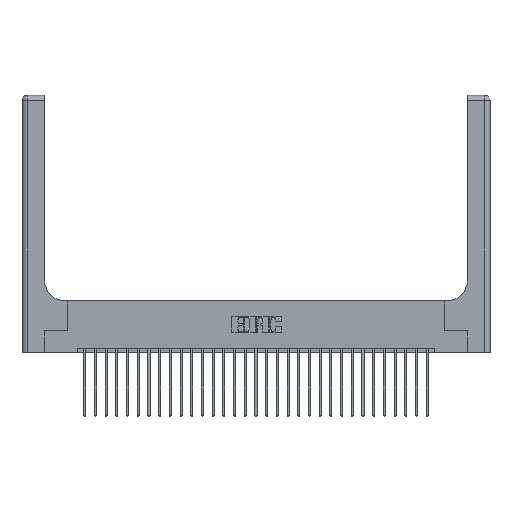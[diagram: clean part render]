
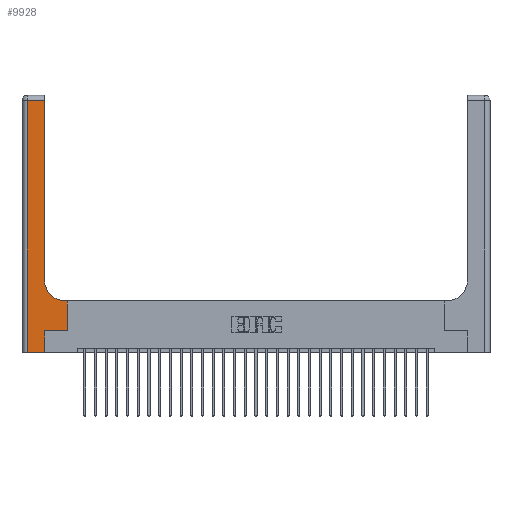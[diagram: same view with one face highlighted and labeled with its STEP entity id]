
A CAD part, top view. The second image highlights one B-rep face of the part: STEP entity #9928.
In plain terms, the highlighted planar face has unit normal (0, 0, 1).
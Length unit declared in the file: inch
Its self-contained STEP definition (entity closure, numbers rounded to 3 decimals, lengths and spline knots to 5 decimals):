
#800 = DIRECTION ( 'NONE',  ( 0., 1., 0. ) ) ;
#1074 = CARTESIAN_POINT ( 'NONE',  ( 0.51, 0.6, 0.37 ) ) ;
#1506 = ORIENTED_EDGE ( 'NONE', *, *, #21290, .T. ) ;
#2542 = CARTESIAN_POINT ( 'NONE',  ( 0.528, 0.25, 0.37 ) ) ;
#5061 = CARTESIAN_POINT ( 'NONE',  ( 0.51, 0.85, 0.37 ) ) ;
#5856 = CARTESIAN_POINT ( 'NONE',  ( 0., 0., 0.37 ) ) ;
#5992 = LINE ( 'NONE', #14007, #18834 ) ;
#6146 = DIRECTION ( 'NONE',  ( 1., 0., 0. ) ) ;
#6627 = ORIENTED_EDGE ( 'NONE', *, *, #27647, .T. ) ;
#6650 = DIRECTION ( 'NONE',  ( 0., 1., 0. ) ) ;
#7171 = VECTOR ( 'NONE', #800, 39.37008 ) ;
#7506 = CARTESIAN_POINT ( 'NONE',  ( 0.26, 2.94, 0.37 ) ) ;
#7764 = ORIENTED_EDGE ( 'NONE', *, *, #26584, .T. ) ;
#7914 = CARTESIAN_POINT ( 'NONE',  ( 0.06, 0., 0.37 ) ) ;
#8118 = DIRECTION ( 'NONE',  ( 0., 0., -1. ) ) ;
#9003 = CARTESIAN_POINT ( 'NONE',  ( 0.26, 3., 0.37 ) ) ;
#9518 = LINE ( 'NONE', #13401, #7171 ) ;
#9928 = ADVANCED_FACE ( 'NONE', ( #19745 ), #16728, .F. ) ;
#9992 = AXIS2_PLACEMENT_3D ( 'NONE', #23475, #8118, #25676 ) ;
#11056 = CARTESIAN_POINT ( 'NONE',  ( 0.265, 0.25, 0.37 ) ) ;
#11061 = VERTEX_POINT ( 'NONE', #2542 ) ;
#11272 = CARTESIAN_POINT ( 'NONE',  ( 0.528, 0.6, 0.37 ) ) ;
#11327 = ORIENTED_EDGE ( 'NONE', *, *, #14260, .T. ) ;
#11352 = CARTESIAN_POINT ( 'NONE',  ( 0.265, 0.25, 0.37 ) ) ;
#11726 = DIRECTION ( 'NONE',  ( 0., -1., 0. ) ) ;
#11970 = EDGE_CURVE ( 'NONE', #19686, #14375, #26737, .T. ) ;
#12166 = VERTEX_POINT ( 'NONE', #1074 ) ;
#13065 = ORIENTED_EDGE ( 'NONE', *, *, #27067, .T. ) ;
#13116 = VERTEX_POINT ( 'NONE', #19005 ) ;
#13401 = CARTESIAN_POINT ( 'NONE',  ( 0.528, 0.25, 0.37 ) ) ;
#13764 = DIRECTION ( 'NONE',  ( 1., 0., 0. ) ) ;
#13942 = LINE ( 'NONE', #11056, #23714 ) ;
#14007 = CARTESIAN_POINT ( 'NONE',  ( 0.06, 3., 0.37 ) ) ;
#14113 = VERTEX_POINT ( 'NONE', #27841 ) ;
#14260 = EDGE_CURVE ( 'NONE', #23562, #11061, #13942, .T. ) ;
#14375 = VERTEX_POINT ( 'NONE', #24067 ) ;
#15113 = VERTEX_POINT ( 'NONE', #11272 ) ;
#15201 = EDGE_LOOP ( 'NONE', ( #25582, #21478, #20221, #13065, #6627, #11327, #1506, #7764, #18355 ) ) ;
#16451 = CIRCLE ( 'NONE', #16591, 0.25 ) ;
#16591 = AXIS2_PLACEMENT_3D ( 'NONE', #5061, #20180, #13764 ) ;
#16728 = PLANE ( 'NONE',  #9992 ) ;
#16998 = VECTOR ( 'NONE', #6650, 39.37008 ) ;
#17060 = LINE ( 'NONE', #25092, #20072 ) ;
#17682 = DIRECTION ( 'NONE',  ( 1., 0., 0. ) ) ;
#17810 = DIRECTION ( 'NONE',  ( 0., 1., 0. ) ) ;
#18355 = ORIENTED_EDGE ( 'NONE', *, *, #24389, .T. ) ;
#18834 = VECTOR ( 'NONE', #11726, 39.37008 ) ;
#19005 = CARTESIAN_POINT ( 'NONE',  ( 0.26, 0.85, 0.37 ) ) ;
#19288 = DIRECTION ( 'NONE',  ( -1., 0., 0. ) ) ;
#19499 = VECTOR ( 'NONE', #6146, 39.37008 ) ;
#19686 = VERTEX_POINT ( 'NONE', #7506 ) ;
#19745 = FACE_OUTER_BOUND ( 'NONE', #15201, .T. ) ;
#20072 = VECTOR ( 'NONE', #25000, 39.37008 ) ;
#20180 = DIRECTION ( 'NONE',  ( 0., 0., -1. ) ) ;
#20221 = ORIENTED_EDGE ( 'NONE', *, *, #23739, .T. ) ;
#20867 = EDGE_CURVE ( 'NONE', #13116, #19686, #22048, .T. ) ;
#21290 = EDGE_CURVE ( 'NONE', #11061, #15113, #9518, .T. ) ;
#21478 = ORIENTED_EDGE ( 'NONE', *, *, #11970, .T. ) ;
#21532 = LINE ( 'NONE', #26359, #27582 ) ;
#21968 = VERTEX_POINT ( 'NONE', #7914 ) ;
#22048 = LINE ( 'NONE', #9003, #16998 ) ;
#23475 = CARTESIAN_POINT ( 'NONE',  ( 0., 3., 0.37 ) ) ;
#23562 = VERTEX_POINT ( 'NONE', #11352 ) ;
#23714 = VECTOR ( 'NONE', #17682, 39.37008 ) ;
#23739 = EDGE_CURVE ( 'NONE', #14375, #21968, #5992, .T. ) ;
#24067 = CARTESIAN_POINT ( 'NONE',  ( 0.06, 2.94, 0.37 ) ) ;
#24389 = EDGE_CURVE ( 'NONE', #12166, #13116, #16451, .T. ) ;
#25000 = DIRECTION ( 'NONE',  ( -1., 0., 0. ) ) ;
#25092 = CARTESIAN_POINT ( 'NONE',  ( 0.26, 0.6, 0.37 ) ) ;
#25247 = LINE ( 'NONE', #5856, #19499 ) ;
#25582 = ORIENTED_EDGE ( 'NONE', *, *, #20867, .T. ) ;
#25676 = DIRECTION ( 'NONE',  ( -1., 0., 0. ) ) ;
#25701 = CARTESIAN_POINT ( 'NONE',  ( 0., 2.94, 0.37 ) ) ;
#26359 = CARTESIAN_POINT ( 'NONE',  ( 0.265, 0., 0.37 ) ) ;
#26423 = VECTOR ( 'NONE', #19288, 39.37008 ) ;
#26584 = EDGE_CURVE ( 'NONE', #15113, #12166, #17060, .T. ) ;
#26737 = LINE ( 'NONE', #25701, #26423 ) ;
#27067 = EDGE_CURVE ( 'NONE', #21968, #14113, #25247, .T. ) ;
#27582 = VECTOR ( 'NONE', #17810, 39.37008 ) ;
#27647 = EDGE_CURVE ( 'NONE', #14113, #23562, #21532, .T. ) ;
#27841 = CARTESIAN_POINT ( 'NONE',  ( 0.265, 0., 0.37 ) ) ;
